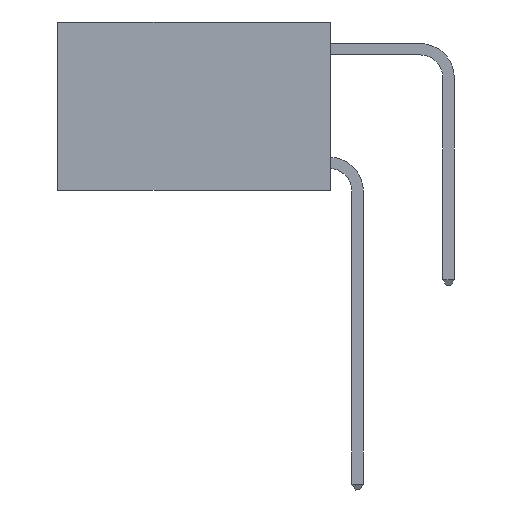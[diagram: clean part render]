
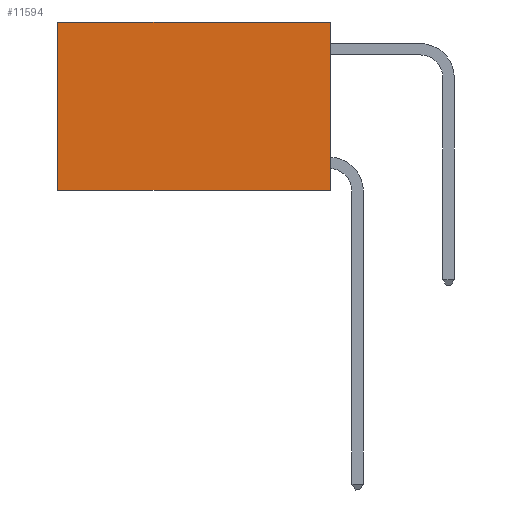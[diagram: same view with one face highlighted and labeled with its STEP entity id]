
A CAD part, left-side view. The second image highlights one B-rep face of the part: STEP entity #11594.
In plain terms, the highlighted planar face has unit normal (-1, 0, 0).
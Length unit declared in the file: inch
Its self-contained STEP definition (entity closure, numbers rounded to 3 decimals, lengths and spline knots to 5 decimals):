
#40 = ORIENTED_EDGE ( 'NONE', *, *, #7379, .T. ) ;
#320 = VECTOR ( 'NONE', #11585, 39.37008 ) ;
#329 = LINE ( 'NONE', #4663, #320 ) ;
#1199 = ORIENTED_EDGE ( 'NONE', *, *, #5957, .F. ) ;
#1344 = CARTESIAN_POINT ( 'NONE',  ( 0.2625, 0., 0. ) ) ;
#1648 = EDGE_CURVE ( 'NONE', #2435, #7485, #329, .T. ) ;
#2185 = CARTESIAN_POINT ( 'NONE',  ( 0.2625, 0., 0. ) ) ;
#2209 = DIRECTION ( 'NONE',  ( 0., 1., 0. ) ) ;
#2430 = LINE ( 'NONE', #10394, #11570 ) ;
#2435 = VERTEX_POINT ( 'NONE', #11096 ) ;
#2682 = VERTEX_POINT ( 'NONE', #8889 ) ;
#2695 = VERTEX_POINT ( 'NONE', #5309 ) ;
#3421 = DIRECTION ( 'NONE',  ( 0., 0., -1. ) ) ;
#3857 = EDGE_CURVE ( 'NONE', #2435, #2695, #10870, .T. ) ;
#4329 = EDGE_LOOP ( 'NONE', ( #40, #1199, #8660, #10134 ) ) ;
#4663 = CARTESIAN_POINT ( 'NONE',  ( 0.2625, 0., 0. ) ) ;
#4898 = FACE_OUTER_BOUND ( 'NONE', #4329, .T. ) ;
#5032 = DIRECTION ( 'NONE',  ( 0., 1., 0. ) ) ;
#5309 = CARTESIAN_POINT ( 'NONE',  ( 0.2625, 0.6, 0. ) ) ;
#5957 = EDGE_CURVE ( 'NONE', #7485, #2682, #2430, .T. ) ;
#5984 = DIRECTION ( 'NONE',  ( 0., 0., -1. ) ) ;
#6293 = CARTESIAN_POINT ( 'NONE',  ( 0.2625, 0., -0.37 ) ) ;
#6411 = VECTOR ( 'NONE', #3421, 39.37008 ) ;
#7379 = EDGE_CURVE ( 'NONE', #2695, #2682, #11041, .T. ) ;
#7485 = VERTEX_POINT ( 'NONE', #6293 ) ;
#8319 = VECTOR ( 'NONE', #2209, 39.37008 ) ;
#8660 = ORIENTED_EDGE ( 'NONE', *, *, #1648, .F. ) ;
#8889 = CARTESIAN_POINT ( 'NONE',  ( 0.2625, 0.6, -0.37 ) ) ;
#8896 = AXIS2_PLACEMENT_3D ( 'NONE', #1344, #11220, #5984 ) ;
#9663 = CARTESIAN_POINT ( 'NONE',  ( 0.2625, 0.6, 0. ) ) ;
#10134 = ORIENTED_EDGE ( 'NONE', *, *, #3857, .T. ) ;
#10394 = CARTESIAN_POINT ( 'NONE',  ( 0.2625, 0., -0.37 ) ) ;
#10870 = LINE ( 'NONE', #2185, #8319 ) ;
#11041 = LINE ( 'NONE', #9663, #6411 ) ;
#11096 = CARTESIAN_POINT ( 'NONE',  ( 0.2625, 0., 0. ) ) ;
#11186 = PLANE ( 'NONE',  #8896 ) ;
#11220 = DIRECTION ( 'NONE',  ( 1., 0., 0. ) ) ;
#11570 = VECTOR ( 'NONE', #5032, 39.37008 ) ;
#11585 = DIRECTION ( 'NONE',  ( 0., 0., -1. ) ) ;
#11594 = ADVANCED_FACE ( 'NONE', ( #4898 ), #11186, .F. ) ;
